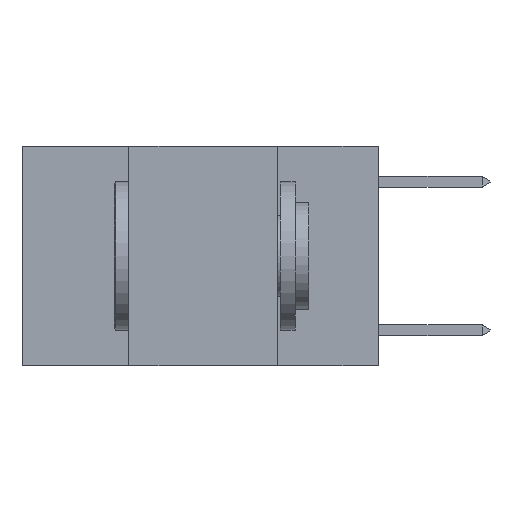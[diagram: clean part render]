
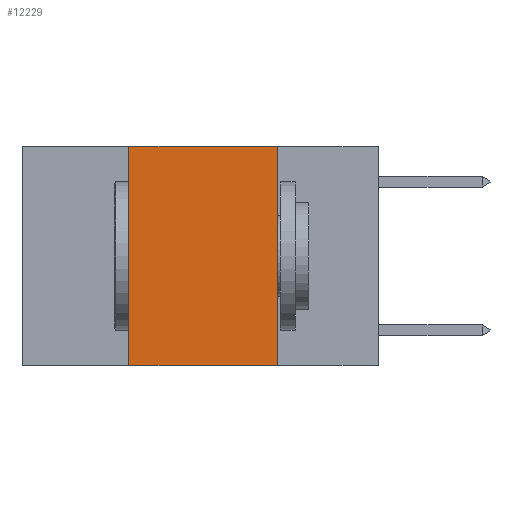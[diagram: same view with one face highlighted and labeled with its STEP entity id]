
A CAD part, left-side view. The second image highlights one B-rep face of the part: STEP entity #12229.
In plain terms, the highlighted planar face has unit normal (-1, 0, 0).
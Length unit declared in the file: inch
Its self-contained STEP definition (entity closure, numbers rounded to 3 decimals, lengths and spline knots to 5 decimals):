
#11 = FACE_OUTER_BOUND ( 'NONE', #14360, .T. ) ;
#332 = ORIENTED_EDGE ( 'NONE', *, *, #28184, .F. ) ;
#710 = CARTESIAN_POINT ( 'NONE',  ( 0., 0.17, 0. ) ) ;
#890 = VECTOR ( 'NONE', #4735, 39.37008 ) ;
#2522 = LINE ( 'NONE', #14127, #19120 ) ;
#3904 = DIRECTION ( 'NONE',  ( 0., -1., 0. ) ) ;
#4511 = VECTOR ( 'NONE', #12938, 39.37008 ) ;
#4735 = DIRECTION ( 'NONE',  ( 0., -1., 0. ) ) ;
#5587 = LINE ( 'NONE', #26638, #18895 ) ;
#7168 = ORIENTED_EDGE ( 'NONE', *, *, #17196, .F. ) ;
#8654 = CARTESIAN_POINT ( 'NONE',  ( 0., 0.6, 0. ) ) ;
#9222 = VERTEX_POINT ( 'NONE', #28003 ) ;
#11021 = DIRECTION ( 'NONE',  ( 0., 0., -1. ) ) ;
#11804 = EDGE_CURVE ( 'NONE', #9222, #18737, #27766, .T. ) ;
#12229 = ADVANCED_FACE ( 'NONE', ( #11 ), #20341, .F. ) ;
#12938 = DIRECTION ( 'NONE',  ( 0., 0., 1. ) ) ;
#13277 = DIRECTION ( 'NONE',  ( 1., 0., 0. ) ) ;
#14127 = CARTESIAN_POINT ( 'NONE',  ( 0., 0.17, 0. ) ) ;
#14360 = EDGE_LOOP ( 'NONE', ( #332, #7168, #29462, #27000 ) ) ;
#14970 = VERTEX_POINT ( 'NONE', #15456 ) ;
#15456 = CARTESIAN_POINT ( 'NONE',  ( 0., 0.42, 0. ) ) ;
#15720 = EDGE_CURVE ( 'NONE', #9222, #14970, #21937, .T. ) ;
#17196 = EDGE_CURVE ( 'NONE', #14970, #20780, #5587, .T. ) ;
#18737 = VERTEX_POINT ( 'NONE', #28782 ) ;
#18895 = VECTOR ( 'NONE', #3904, 39.37008 ) ;
#19120 = VECTOR ( 'NONE', #23752, 39.37008 ) ;
#20341 = PLANE ( 'NONE',  #22060 ) ;
#20780 = VERTEX_POINT ( 'NONE', #710 ) ;
#21777 = CARTESIAN_POINT ( 'NONE',  ( 0., 0.42, 0. ) ) ;
#21937 = LINE ( 'NONE', #21777, #4511 ) ;
#22060 = AXIS2_PLACEMENT_3D ( 'NONE', #8654, #13277, #11021 ) ;
#23752 = DIRECTION ( 'NONE',  ( 0., 0., -1. ) ) ;
#26638 = CARTESIAN_POINT ( 'NONE',  ( 0., 0.6, 0. ) ) ;
#27000 = ORIENTED_EDGE ( 'NONE', *, *, #11804, .T. ) ;
#27469 = CARTESIAN_POINT ( 'NONE',  ( 0., 0.6, -0.37 ) ) ;
#27766 = LINE ( 'NONE', #27469, #890 ) ;
#28003 = CARTESIAN_POINT ( 'NONE',  ( 0., 0.42, -0.37 ) ) ;
#28184 = EDGE_CURVE ( 'NONE', #20780, #18737, #2522, .T. ) ;
#28782 = CARTESIAN_POINT ( 'NONE',  ( 0., 0.17, -0.37 ) ) ;
#29462 = ORIENTED_EDGE ( 'NONE', *, *, #15720, .F. ) ;
